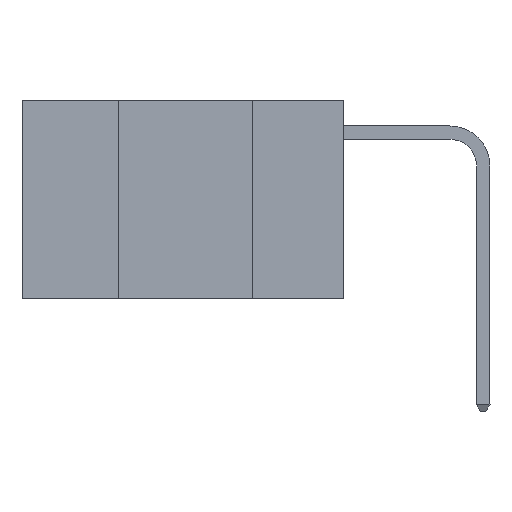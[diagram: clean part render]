
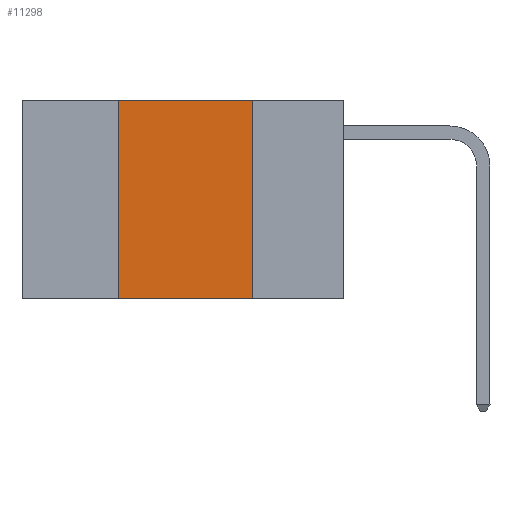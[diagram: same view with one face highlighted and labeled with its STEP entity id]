
A CAD part, left-side view. The second image highlights one B-rep face of the part: STEP entity #11298.
In plain terms, the highlighted planar face has unit normal (-1, 0, 0).
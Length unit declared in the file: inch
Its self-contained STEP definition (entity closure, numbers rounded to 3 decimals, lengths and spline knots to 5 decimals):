
#503 = LINE ( 'NONE', #2532, #12413 ) ;
#1767 = ORIENTED_EDGE ( 'NONE', *, *, #10339, .F. ) ;
#1861 = ORIENTED_EDGE ( 'NONE', *, *, #4437, .F. ) ;
#1871 = ORIENTED_EDGE ( 'NONE', *, *, #6418, .F. ) ;
#2120 = VECTOR ( 'NONE', #6625, 39.37008 ) ;
#2242 = LINE ( 'NONE', #6577, #2120 ) ;
#2264 = ORIENTED_EDGE ( 'NONE', *, *, #7508, .T. ) ;
#2532 = CARTESIAN_POINT ( 'NONE',  ( 0., 0.6, 0. ) ) ;
#3198 = CARTESIAN_POINT ( 'NONE',  ( 0., 0.17, 0. ) ) ;
#4402 = DIRECTION ( 'NONE',  ( 0., 0., -1. ) ) ;
#4437 = EDGE_CURVE ( 'NONE', #8789, #9152, #7186, .T. ) ;
#4758 = DIRECTION ( 'NONE',  ( 0., -1., 0. ) ) ;
#4859 = CARTESIAN_POINT ( 'NONE',  ( 0., 0.6, -0.37 ) ) ;
#6375 = CARTESIAN_POINT ( 'NONE',  ( 0., 0.42, 0. ) ) ;
#6385 = EDGE_LOOP ( 'NONE', ( #1861, #1767, #1871, #2264 ) ) ;
#6418 = EDGE_CURVE ( 'NONE', #9083, #8810, #2242, .T. ) ;
#6577 = CARTESIAN_POINT ( 'NONE',  ( 0., 0.42, 0. ) ) ;
#6625 = DIRECTION ( 'NONE',  ( 0., 0., 1. ) ) ;
#6764 = DIRECTION ( 'NONE',  ( 0., -1., 0. ) ) ;
#7174 = VECTOR ( 'NONE', #8782, 39.37008 ) ;
#7186 = LINE ( 'NONE', #8775, #7174 ) ;
#7508 = EDGE_CURVE ( 'NONE', #9083, #9152, #8431, .T. ) ;
#8431 = LINE ( 'NONE', #4859, #8623 ) ;
#8623 = VECTOR ( 'NONE', #4758, 39.37008 ) ;
#8775 = CARTESIAN_POINT ( 'NONE',  ( 0., 0.17, 0. ) ) ;
#8782 = DIRECTION ( 'NONE',  ( 0., 0., -1. ) ) ;
#8789 = VERTEX_POINT ( 'NONE', #3198 ) ;
#8810 = VERTEX_POINT ( 'NONE', #6375 ) ;
#9034 = AXIS2_PLACEMENT_3D ( 'NONE', #9411, #10435, #4402 ) ;
#9083 = VERTEX_POINT ( 'NONE', #9774 ) ;
#9152 = VERTEX_POINT ( 'NONE', #9900 ) ;
#9411 = CARTESIAN_POINT ( 'NONE',  ( 0., 0.6, 0. ) ) ;
#9774 = CARTESIAN_POINT ( 'NONE',  ( 0., 0.42, -0.37 ) ) ;
#9900 = CARTESIAN_POINT ( 'NONE',  ( 0., 0.17, -0.37 ) ) ;
#10339 = EDGE_CURVE ( 'NONE', #8810, #8789, #503, .T. ) ;
#10384 = PLANE ( 'NONE',  #9034 ) ;
#10435 = DIRECTION ( 'NONE',  ( 1., 0., 0. ) ) ;
#10634 = FACE_OUTER_BOUND ( 'NONE', #6385, .T. ) ;
#11298 = ADVANCED_FACE ( 'NONE', ( #10634 ), #10384, .F. ) ;
#12413 = VECTOR ( 'NONE', #6764, 39.37008 ) ;
